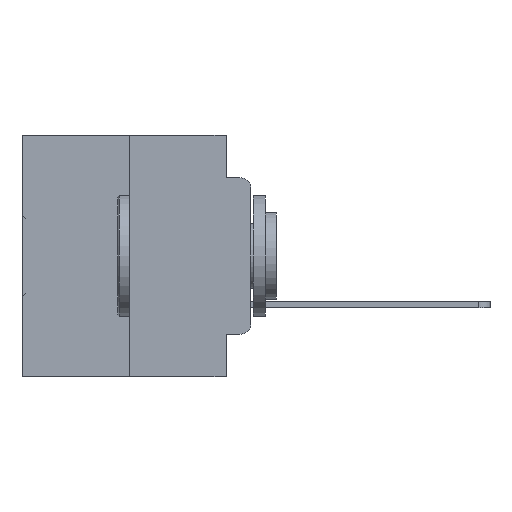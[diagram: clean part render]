
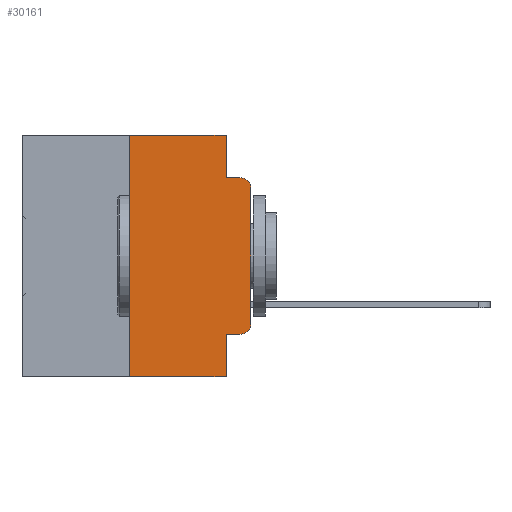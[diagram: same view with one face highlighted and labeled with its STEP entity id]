
A CAD part, left-side view. The second image highlights one B-rep face of the part: STEP entity #30161.
In plain terms, the highlighted planar face has unit normal (-1, 0, 0).
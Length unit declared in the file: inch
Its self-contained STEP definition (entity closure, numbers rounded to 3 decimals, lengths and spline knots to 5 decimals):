
#2428 = LINE ( 'NONE', #5720, #7314 ) ;
#2788 = CARTESIAN_POINT ( 'NONE',  ( 0., 0.051, -0.4115 ) ) ;
#2921 = EDGE_CURVE ( 'NONE', #20576, #7808, #2428, .T. ) ;
#3273 = VECTOR ( 'NONE', #8013, 39.37008 ) ;
#4113 = VECTOR ( 'NONE', #30062, 39.37008 ) ;
#4170 = LINE ( 'NONE', #21547, #3273 ) ;
#4543 = EDGE_CURVE ( 'NONE', #29008, #26616, #24220, .T. ) ;
#4613 = VERTEX_POINT ( 'NONE', #15041 ) ;
#5270 = CARTESIAN_POINT ( 'NONE',  ( 0., 0., -0.1085 ) ) ;
#5657 = LINE ( 'NONE', #26885, #32978 ) ;
#5705 = ORIENTED_EDGE ( 'NONE', *, *, #19938, .T. ) ;
#5720 = CARTESIAN_POINT ( 'NONE',  ( 0., 0.473, -0.5 ) ) ;
#6434 = EDGE_CURVE ( 'NONE', #24531, #26616, #30799, .T. ) ;
#7062 = DIRECTION ( 'NONE',  ( -1., 0., 0. ) ) ;
#7314 = VECTOR ( 'NONE', #22062, 39.37008 ) ;
#7808 = VERTEX_POINT ( 'NONE', #29138 ) ;
#7965 = CARTESIAN_POINT ( 'NONE',  ( 0., 0., 0. ) ) ;
#8013 = DIRECTION ( 'NONE',  ( 0., 0., -1. ) ) ;
#8233 = DIRECTION ( 'NONE',  ( 0., 0., 1. ) ) ;
#8350 = EDGE_CURVE ( 'NONE', #4613, #24531, #28686, .T. ) ;
#8360 = ORIENTED_EDGE ( 'NONE', *, *, #28585, .F. ) ;
#9227 = CARTESIAN_POINT ( 'NONE',  ( 0., 0.25, -0.5 ) ) ;
#9596 = PLANE ( 'NONE',  #11880 ) ;
#9971 = CARTESIAN_POINT ( 'NONE',  ( 0., 0.051, 0. ) ) ;
#11766 = CARTESIAN_POINT ( 'NONE',  ( 0., 0.473, 0. ) ) ;
#11819 = CARTESIAN_POINT ( 'NONE',  ( 0., 0.051, -0.4115 ) ) ;
#11880 = AXIS2_PLACEMENT_3D ( 'NONE', #27982, #28088, #12445 ) ;
#12445 = DIRECTION ( 'NONE',  ( 0., 0., -1. ) ) ;
#13149 = DIRECTION ( 'NONE',  ( -1., 0., 0. ) ) ;
#14445 = DIRECTION ( 'NONE',  ( 0., -1., 0. ) ) ;
#14726 = VERTEX_POINT ( 'NONE', #22527 ) ;
#15041 = CARTESIAN_POINT ( 'NONE',  ( 0., 0., -0.3915 ) ) ;
#15517 = CARTESIAN_POINT ( 'NONE',  ( 0., 0.051, -0.0885 ) ) ;
#15572 = CARTESIAN_POINT ( 'NONE',  ( 0., 0.051, 0. ) ) ;
#15631 = VECTOR ( 'NONE', #31603, 39.37008 ) ;
#15674 = ORIENTED_EDGE ( 'NONE', *, *, #18145, .T. ) ;
#15685 = VECTOR ( 'NONE', #14445, 39.37008 ) ;
#15938 = CIRCLE ( 'NONE', #22637, 0.02 ) ;
#16246 = VERTEX_POINT ( 'NONE', #15572 ) ;
#16598 = CARTESIAN_POINT ( 'NONE',  ( 0., 0.02, -0.0885 ) ) ;
#17895 = LINE ( 'NONE', #11819, #4113 ) ;
#18145 = EDGE_CURVE ( 'NONE', #25010, #4613, #15938, .T. ) ;
#19938 = EDGE_CURVE ( 'NONE', #34026, #25010, #17895, .T. ) ;
#20576 = VERTEX_POINT ( 'NONE', #9227 ) ;
#21542 = ORIENTED_EDGE ( 'NONE', *, *, #8350, .T. ) ;
#21547 = CARTESIAN_POINT ( 'NONE',  ( 0., 0.051, 0. ) ) ;
#21721 = EDGE_CURVE ( 'NONE', #34026, #7808, #4170, .T. ) ;
#21836 = LINE ( 'NONE', #9971, #28631 ) ;
#22062 = DIRECTION ( 'NONE',  ( 0., -1., 0. ) ) ;
#22527 = CARTESIAN_POINT ( 'NONE',  ( 0., 0.25, 0. ) ) ;
#22637 = AXIS2_PLACEMENT_3D ( 'NONE', #28774, #13149, #31279 ) ;
#23260 = CARTESIAN_POINT ( 'NONE',  ( 0., 0.02, -0.1085 ) ) ;
#23295 = DIRECTION ( 'NONE',  ( 0., 0., -1. ) ) ;
#23404 = VECTOR ( 'NONE', #30392, 39.37008 ) ;
#24220 = LINE ( 'NONE', #27849, #23404 ) ;
#24257 = FACE_OUTER_BOUND ( 'NONE', #24725, .T. ) ;
#24531 = VERTEX_POINT ( 'NONE', #5270 ) ;
#24725 = EDGE_LOOP ( 'NONE', ( #21542, #31473, #27980, #34285, #32731, #8360, #31050, #24726, #5705, #15674 ) ) ;
#24726 = ORIENTED_EDGE ( 'NONE', *, *, #21721, .F. ) ;
#25010 = VERTEX_POINT ( 'NONE', #33550 ) ;
#25816 = DIRECTION ( 'NONE',  ( 0., 0., -1. ) ) ;
#26616 = VERTEX_POINT ( 'NONE', #16598 ) ;
#26885 = CARTESIAN_POINT ( 'NONE',  ( 0., 0.25, 0. ) ) ;
#27366 = EDGE_CURVE ( 'NONE', #14726, #16246, #29534, .T. ) ;
#27849 = CARTESIAN_POINT ( 'NONE',  ( 0., 0.051, -0.0885 ) ) ;
#27963 = AXIS2_PLACEMENT_3D ( 'NONE', #23260, #7062, #25816 ) ;
#27980 = ORIENTED_EDGE ( 'NONE', *, *, #4543, .F. ) ;
#27982 = CARTESIAN_POINT ( 'NONE',  ( 0., 0.473, 0. ) ) ;
#28088 = DIRECTION ( 'NONE',  ( 1., 0., 0. ) ) ;
#28585 = EDGE_CURVE ( 'NONE', #20576, #14726, #5657, .T. ) ;
#28631 = VECTOR ( 'NONE', #23295, 39.37008 ) ;
#28686 = LINE ( 'NONE', #7965, #15631 ) ;
#28774 = CARTESIAN_POINT ( 'NONE',  ( 0., 0.02, -0.3915 ) ) ;
#29008 = VERTEX_POINT ( 'NONE', #15517 ) ;
#29138 = CARTESIAN_POINT ( 'NONE',  ( 0., 0.051, -0.5 ) ) ;
#29534 = LINE ( 'NONE', #11766, #15685 ) ;
#30062 = DIRECTION ( 'NONE',  ( 0., -1., 0. ) ) ;
#30161 = ADVANCED_FACE ( 'NONE', ( #24257 ), #9596, .F. ) ;
#30276 = EDGE_CURVE ( 'NONE', #16246, #29008, #21836, .T. ) ;
#30392 = DIRECTION ( 'NONE',  ( 0., -1., 0. ) ) ;
#30799 = CIRCLE ( 'NONE', #27963, 0.02 ) ;
#31050 = ORIENTED_EDGE ( 'NONE', *, *, #2921, .T. ) ;
#31279 = DIRECTION ( 'NONE',  ( 0., 0., -1. ) ) ;
#31473 = ORIENTED_EDGE ( 'NONE', *, *, #6434, .T. ) ;
#31603 = DIRECTION ( 'NONE',  ( 0., 0., 1. ) ) ;
#32731 = ORIENTED_EDGE ( 'NONE', *, *, #27366, .F. ) ;
#32978 = VECTOR ( 'NONE', #8233, 39.37008 ) ;
#33550 = CARTESIAN_POINT ( 'NONE',  ( 0., 0.02, -0.4115 ) ) ;
#34026 = VERTEX_POINT ( 'NONE', #2788 ) ;
#34285 = ORIENTED_EDGE ( 'NONE', *, *, #30276, .F. ) ;
